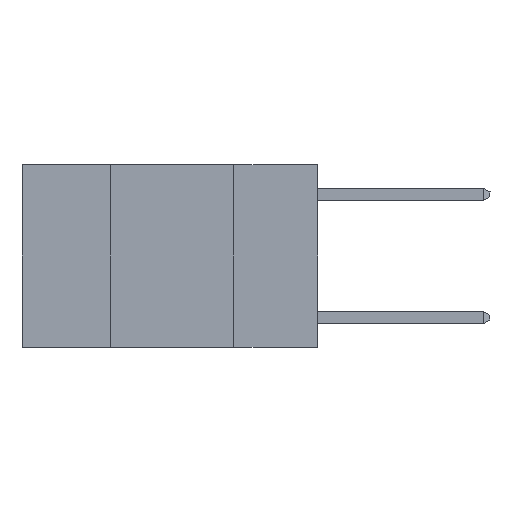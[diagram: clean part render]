
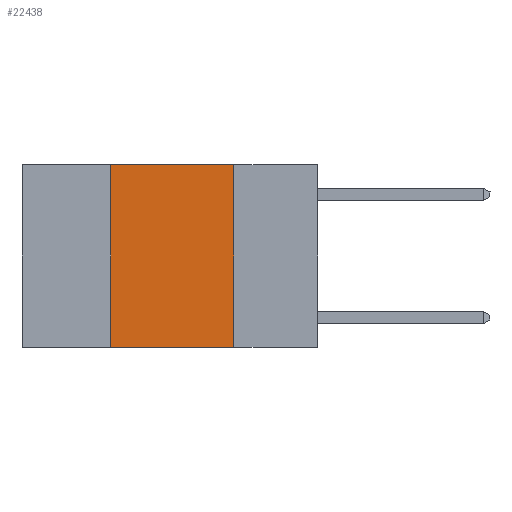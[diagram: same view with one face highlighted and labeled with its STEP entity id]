
A CAD part, left-side view. The second image highlights one B-rep face of the part: STEP entity #22438.
In plain terms, the highlighted planar face has unit normal (-1, 0, 0).
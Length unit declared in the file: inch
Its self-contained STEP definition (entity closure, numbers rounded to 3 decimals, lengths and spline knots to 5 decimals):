
#63 = VECTOR ( 'NONE', #937, 39.37008 ) ;
#539 = AXIS2_PLACEMENT_3D ( 'NONE', #13092, #3976, #23173 ) ;
#937 = DIRECTION ( 'NONE',  ( 0., 0., 1. ) ) ;
#2138 = ORIENTED_EDGE ( 'NONE', *, *, #3522, .F. ) ;
#2586 = CARTESIAN_POINT ( 'NONE',  ( 0., 0.6, 0. ) ) ;
#3522 = EDGE_CURVE ( 'NONE', #18840, #5602, #8643, .T. ) ;
#3887 = VECTOR ( 'NONE', #6537, 39.37008 ) ;
#3976 = DIRECTION ( 'NONE',  ( 1., 0., 0. ) ) ;
#4337 = ORIENTED_EDGE ( 'NONE', *, *, #10345, .F. ) ;
#4510 = CARTESIAN_POINT ( 'NONE',  ( 0., 0.17, 0. ) ) ;
#4531 = FACE_OUTER_BOUND ( 'NONE', #22012, .T. ) ;
#5602 = VERTEX_POINT ( 'NONE', #5851 ) ;
#5851 = CARTESIAN_POINT ( 'NONE',  ( 0., 0.17, 0. ) ) ;
#6537 = DIRECTION ( 'NONE',  ( 0., 0., -1. ) ) ;
#8574 = VECTOR ( 'NONE', #13414, 39.37008 ) ;
#8643 = LINE ( 'NONE', #2586, #16412 ) ;
#8899 = CARTESIAN_POINT ( 'NONE',  ( 0., 0.42, 0. ) ) ;
#9538 = ORIENTED_EDGE ( 'NONE', *, *, #23968, .T. ) ;
#10345 = EDGE_CURVE ( 'NONE', #15312, #18840, #12798, .T. ) ;
#11324 = ORIENTED_EDGE ( 'NONE', *, *, #21368, .F. ) ;
#12241 = PLANE ( 'NONE',  #539 ) ;
#12301 = DIRECTION ( 'NONE',  ( 0., -1., 0. ) ) ;
#12798 = LINE ( 'NONE', #16329, #63 ) ;
#13092 = CARTESIAN_POINT ( 'NONE',  ( 0., 0.6, 0. ) ) ;
#13414 = DIRECTION ( 'NONE',  ( 0., -1., 0. ) ) ;
#13941 = VERTEX_POINT ( 'NONE', #20487 ) ;
#15312 = VERTEX_POINT ( 'NONE', #22267 ) ;
#16329 = CARTESIAN_POINT ( 'NONE',  ( 0., 0.42, 0. ) ) ;
#16412 = VECTOR ( 'NONE', #12301, 39.37008 ) ;
#18840 = VERTEX_POINT ( 'NONE', #8899 ) ;
#20487 = CARTESIAN_POINT ( 'NONE',  ( 0., 0.17, -0.37 ) ) ;
#20748 = LINE ( 'NONE', #24656, #8574 ) ;
#21368 = EDGE_CURVE ( 'NONE', #5602, #13941, #21808, .T. ) ;
#21808 = LINE ( 'NONE', #4510, #3887 ) ;
#22012 = EDGE_LOOP ( 'NONE', ( #11324, #2138, #4337, #9538 ) ) ;
#22267 = CARTESIAN_POINT ( 'NONE',  ( 0., 0.42, -0.37 ) ) ;
#22438 = ADVANCED_FACE ( 'NONE', ( #4531 ), #12241, .F. ) ;
#23173 = DIRECTION ( 'NONE',  ( 0., 0., -1. ) ) ;
#23968 = EDGE_CURVE ( 'NONE', #15312, #13941, #20748, .T. ) ;
#24656 = CARTESIAN_POINT ( 'NONE',  ( 0., 0.6, -0.37 ) ) ;
